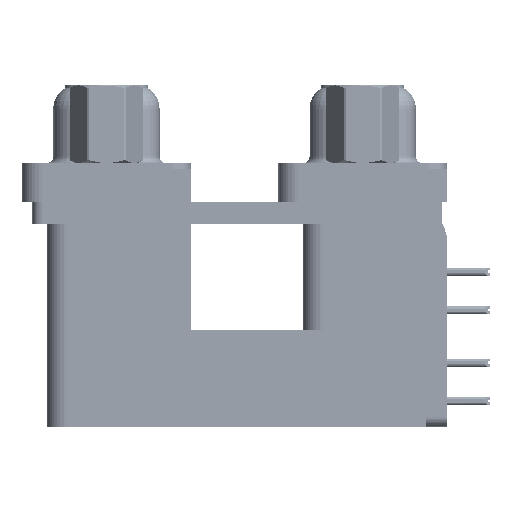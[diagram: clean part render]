
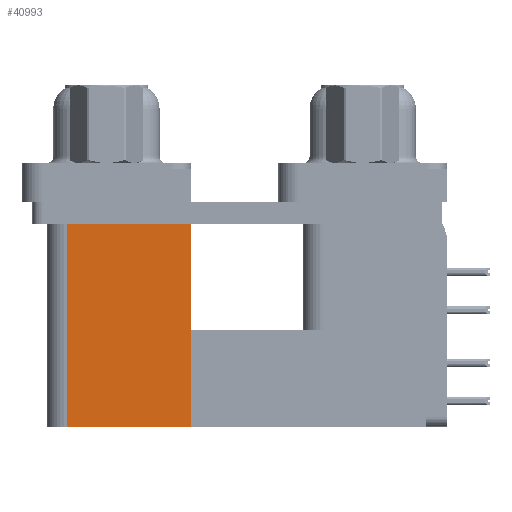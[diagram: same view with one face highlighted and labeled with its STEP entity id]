
A CAD part, left-side view. The second image highlights one B-rep face of the part: STEP entity #40993.
In plain terms, the highlighted planar face has unit normal (-1, 0, 0).
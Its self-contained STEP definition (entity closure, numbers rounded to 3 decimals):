
#1025 = DIRECTION ( 'NONE',  ( 0., 0., 1. ) ) ;
#3483 = CARTESIAN_POINT ( 'NONE',  ( 3.7, 21.975, -19.2 ) ) ;
#4292 = EDGE_CURVE ( 'NONE', #54454, #60421, #28053, .T. ) ;
#8132 = LINE ( 'NONE', #3483, #52195 ) ;
#13589 = DIRECTION ( 'NONE',  ( 0., 1., 0. ) ) ;
#16854 = VECTOR ( 'NONE', #1025, 1000. ) ;
#17675 = EDGE_CURVE ( 'NONE', #57852, #60421, #8132, .T. ) ;
#20411 = EDGE_LOOP ( 'NONE', ( #41679, #45321, #29814, #46402 ) ) ;
#20867 = CARTESIAN_POINT ( 'NONE',  ( 3.7, 12.775, -2.5 ) ) ;
#22693 = DIRECTION ( 'NONE',  ( 0., 0., 1. ) ) ;
#23675 = VECTOR ( 'NONE', #41635, 1000. ) ;
#28053 = LINE ( 'NONE', #20867, #23675 ) ;
#29814 = ORIENTED_EDGE ( 'NONE', *, *, #36609, .F. ) ;
#32259 = DIRECTION ( 'NONE',  ( 0., 1., 0. ) ) ;
#33749 = DIRECTION ( 'NONE',  ( 1., 0., 0. ) ) ;
#36283 = CARTESIAN_POINT ( 'NONE',  ( 3.7, 21.975, -2.5 ) ) ;
#36609 = EDGE_CURVE ( 'NONE', #54669, #57852, #42464, .T. ) ;
#37874 = CARTESIAN_POINT ( 'NONE',  ( 3.7, 12.775, -19.2 ) ) ;
#38327 = CARTESIAN_POINT ( 'NONE',  ( 3.7, 12.775, -2.5 ) ) ;
#38375 = FACE_OUTER_BOUND ( 'NONE', #20411, .T. ) ;
#40043 = EDGE_CURVE ( 'NONE', #54669, #54454, #46286, .T. ) ;
#40993 = ADVANCED_FACE ( 'NONE', ( #38375 ), #63459, .F. ) ;
#41635 = DIRECTION ( 'NONE',  ( 0., 1., 0. ) ) ;
#41645 = CARTESIAN_POINT ( 'NONE',  ( 3.7, 12.775, -19.2 ) ) ;
#41679 = ORIENTED_EDGE ( 'NONE', *, *, #4292, .T. ) ;
#42464 = LINE ( 'NONE', #37874, #61942 ) ;
#45321 = ORIENTED_EDGE ( 'NONE', *, *, #17675, .F. ) ;
#46286 = LINE ( 'NONE', #41645, #16854 ) ;
#46402 = ORIENTED_EDGE ( 'NONE', *, *, #40043, .T. ) ;
#50122 = CARTESIAN_POINT ( 'NONE',  ( 3.7, 12.775, -19.2 ) ) ;
#52195 = VECTOR ( 'NONE', #22693, 1000. ) ;
#53252 = CARTESIAN_POINT ( 'NONE',  ( 3.7, 21.975, -19.2 ) ) ;
#53539 = CARTESIAN_POINT ( 'NONE',  ( 3.7, 12.775, -19.2 ) ) ;
#54454 = VERTEX_POINT ( 'NONE', #38327 ) ;
#54669 = VERTEX_POINT ( 'NONE', #50122 ) ;
#57852 = VERTEX_POINT ( 'NONE', #53252 ) ;
#60421 = VERTEX_POINT ( 'NONE', #36283 ) ;
#61942 = VECTOR ( 'NONE', #32259, 1000. ) ;
#62318 = AXIS2_PLACEMENT_3D ( 'NONE', #53539, #33749, #13589 ) ;
#63459 = PLANE ( 'NONE',  #62318 ) ;
